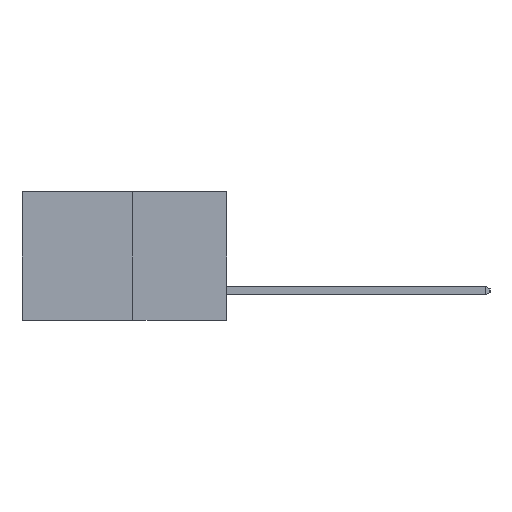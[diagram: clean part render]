
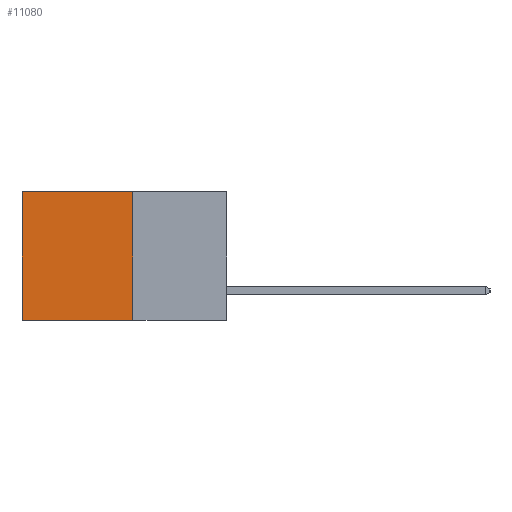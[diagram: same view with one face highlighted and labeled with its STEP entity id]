
A CAD part, left-side view. The second image highlights one B-rep face of the part: STEP entity #11080.
In plain terms, the highlighted planar face has unit normal (-1, 0, 0).
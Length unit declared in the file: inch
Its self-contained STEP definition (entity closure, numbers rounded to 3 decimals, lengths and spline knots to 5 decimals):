
#28 = EDGE_CURVE ( 'NONE', #3556, #13211, #3735, .T. ) ;
#173 = CARTESIAN_POINT ( 'NONE',  ( 0.277, 0.59, -0.37 ) ) ;
#829 = VECTOR ( 'NONE', #7340, 39.37008 ) ;
#1040 = VERTEX_POINT ( 'NONE', #5489 ) ;
#1340 = PLANE ( 'NONE',  #7192 ) ;
#1668 = FACE_OUTER_BOUND ( 'NONE', #8971, .T. ) ;
#2395 = ORIENTED_EDGE ( 'NONE', *, *, #28, .T. ) ;
#2412 = DIRECTION ( 'NONE',  ( 0., 0., -1. ) ) ;
#3556 = VERTEX_POINT ( 'NONE', #10554 ) ;
#3634 = ORIENTED_EDGE ( 'NONE', *, *, #6918, .F. ) ;
#3735 = LINE ( 'NONE', #4895, #829 ) ;
#3898 = VECTOR ( 'NONE', #6944, 39.37008 ) ;
#4825 = CARTESIAN_POINT ( 'NONE',  ( 0.277, 0.27, -0.37 ) ) ;
#4895 = CARTESIAN_POINT ( 'NONE',  ( 0.277, 0.59, -0.37 ) ) ;
#4923 = LINE ( 'NONE', #8038, #9896 ) ;
#4993 = CARTESIAN_POINT ( 'NONE',  ( 0.277, 0.27, 0. ) ) ;
#5153 = EDGE_CURVE ( 'NONE', #5168, #3556, #9593, .T. ) ;
#5168 = VERTEX_POINT ( 'NONE', #8173 ) ;
#5489 = CARTESIAN_POINT ( 'NONE',  ( 0.277, 0.27, -0.37 ) ) ;
#6918 = EDGE_CURVE ( 'NONE', #1040, #13211, #8840, .T. ) ;
#6944 = DIRECTION ( 'NONE',  ( 0., 1., 0. ) ) ;
#7192 = AXIS2_PLACEMENT_3D ( 'NONE', #12796, #8874, #2412 ) ;
#7340 = DIRECTION ( 'NONE',  ( 0., 0., -1. ) ) ;
#8038 = CARTESIAN_POINT ( 'NONE',  ( 0.277, 0.27, -0.37 ) ) ;
#8173 = CARTESIAN_POINT ( 'NONE',  ( 0.277, 0.27, 0. ) ) ;
#8190 = VECTOR ( 'NONE', #9851, 39.37008 ) ;
#8840 = LINE ( 'NONE', #4825, #8190 ) ;
#8874 = DIRECTION ( 'NONE',  ( 1., 0., 0. ) ) ;
#8971 = EDGE_LOOP ( 'NONE', ( #2395, #3634, #11667, #10146 ) ) ;
#9593 = LINE ( 'NONE', #4993, #3898 ) ;
#9851 = DIRECTION ( 'NONE',  ( 0., 1., 0. ) ) ;
#9896 = VECTOR ( 'NONE', #11123, 39.37008 ) ;
#10026 = EDGE_CURVE ( 'NONE', #5168, #1040, #4923, .T. ) ;
#10146 = ORIENTED_EDGE ( 'NONE', *, *, #5153, .T. ) ;
#10554 = CARTESIAN_POINT ( 'NONE',  ( 0.277, 0.59, 0. ) ) ;
#11080 = ADVANCED_FACE ( 'NONE', ( #1668 ), #1340, .F. ) ;
#11123 = DIRECTION ( 'NONE',  ( 0., 0., -1. ) ) ;
#11667 = ORIENTED_EDGE ( 'NONE', *, *, #10026, .F. ) ;
#12796 = CARTESIAN_POINT ( 'NONE',  ( 0.277, 0.27, -0.37 ) ) ;
#13211 = VERTEX_POINT ( 'NONE', #173 ) ;
